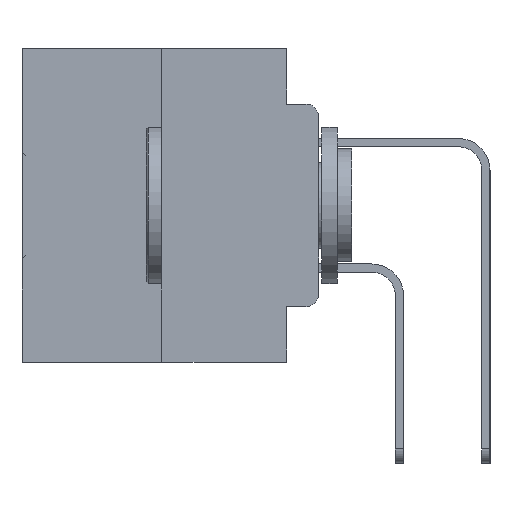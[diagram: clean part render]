
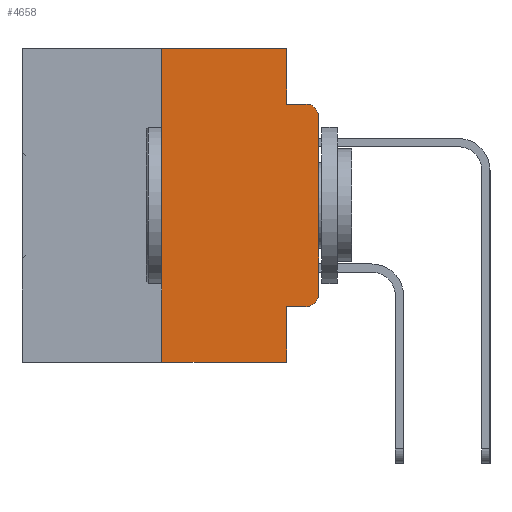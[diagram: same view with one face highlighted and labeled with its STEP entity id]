
A CAD part, left-side view. The second image highlights one B-rep face of the part: STEP entity #4658.
In plain terms, the highlighted planar face has unit normal (-1, 0, 0).
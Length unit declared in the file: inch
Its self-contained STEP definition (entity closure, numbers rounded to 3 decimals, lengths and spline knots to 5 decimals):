
#190 = CARTESIAN_POINT ( 'NONE',  ( 0., 0.473, 0. ) ) ;
#688 = LINE ( 'NONE', #13337, #14145 ) ;
#1972 = EDGE_CURVE ( 'NONE', #3401, #3729, #688, .T. ) ;
#2183 = FACE_OUTER_BOUND ( 'NONE', #27340, .T. ) ;
#2948 = VECTOR ( 'NONE', #24054, 39.37008 ) ;
#3268 = VECTOR ( 'NONE', #16422, 39.37008 ) ;
#3401 = VERTEX_POINT ( 'NONE', #32693 ) ;
#3729 = VERTEX_POINT ( 'NONE', #21136 ) ;
#3745 = DIRECTION ( 'NONE',  ( -1., 0., 0. ) ) ;
#3800 = ORIENTED_EDGE ( 'NONE', *, *, #30094, .T. ) ;
#3919 = CARTESIAN_POINT ( 'NONE',  ( 0., 0.051, -0.4115 ) ) ;
#4105 = AXIS2_PLACEMENT_3D ( 'NONE', #19871, #3745, #22589 ) ;
#4202 = CARTESIAN_POINT ( 'NONE',  ( 0., 0., 0. ) ) ;
#4546 = DIRECTION ( 'NONE',  ( 0., 0., -1. ) ) ;
#4658 = ADVANCED_FACE ( 'NONE', ( #2183 ), #17937, .F. ) ;
#5143 = VERTEX_POINT ( 'NONE', #3919 ) ;
#5626 = CARTESIAN_POINT ( 'NONE',  ( 0., 0.02, -0.4115 ) ) ;
#5742 = EDGE_CURVE ( 'NONE', #5143, #10630, #19257, .T. ) ;
#6447 = LINE ( 'NONE', #190, #11897 ) ;
#6921 = DIRECTION ( 'NONE',  ( 0., 0., 1. ) ) ;
#8018 = ORIENTED_EDGE ( 'NONE', *, *, #17838, .F. ) ;
#8147 = AXIS2_PLACEMENT_3D ( 'NONE', #10281, #29152, #12981 ) ;
#8456 = ORIENTED_EDGE ( 'NONE', *, *, #1972, .F. ) ;
#8635 = CARTESIAN_POINT ( 'NONE',  ( 0., 0.02, -0.0885 ) ) ;
#8859 = VERTEX_POINT ( 'NONE', #20877 ) ;
#8885 = ORIENTED_EDGE ( 'NONE', *, *, #33506, .T. ) ;
#8962 = CARTESIAN_POINT ( 'NONE',  ( 0., 0., -0.3915 ) ) ;
#9283 = EDGE_CURVE ( 'NONE', #5143, #31041, #29585, .T. ) ;
#10090 = LINE ( 'NONE', #34733, #2948 ) ;
#10281 = CARTESIAN_POINT ( 'NONE',  ( 0., 0.02, -0.1085 ) ) ;
#10304 = CARTESIAN_POINT ( 'NONE',  ( 0., 0.051, -0.5 ) ) ;
#10630 = VERTEX_POINT ( 'NONE', #5626 ) ;
#10942 = ORIENTED_EDGE ( 'NONE', *, *, #29273, .T. ) ;
#11369 = ORIENTED_EDGE ( 'NONE', *, *, #27605, .F. ) ;
#11425 = VERTEX_POINT ( 'NONE', #8635 ) ;
#11897 = VECTOR ( 'NONE', #24332, 39.37008 ) ;
#12510 = CARTESIAN_POINT ( 'NONE',  ( 0., 0.473, 0. ) ) ;
#12641 = ORIENTED_EDGE ( 'NONE', *, *, #5742, .T. ) ;
#12981 = DIRECTION ( 'NONE',  ( 0., 0., -1. ) ) ;
#13337 = CARTESIAN_POINT ( 'NONE',  ( 0., 0.25, 0. ) ) ;
#14145 = VECTOR ( 'NONE', #21501, 39.37008 ) ;
#14275 = LINE ( 'NONE', #4202, #27804 ) ;
#14323 = DIRECTION ( 'NONE',  ( 0., -1., 0. ) ) ;
#14712 = CARTESIAN_POINT ( 'NONE',  ( 0., 0.051, 0. ) ) ;
#14745 = CIRCLE ( 'NONE', #8147, 0.02 ) ;
#15294 = EDGE_CURVE ( 'NONE', #34616, #11425, #14745, .T. ) ;
#16422 = DIRECTION ( 'NONE',  ( 0., 0., -1. ) ) ;
#16773 = DIRECTION ( 'NONE',  ( 0., -1., 0. ) ) ;
#16827 = ORIENTED_EDGE ( 'NONE', *, *, #33002, .F. ) ;
#16978 = CARTESIAN_POINT ( 'NONE',  ( 0., 0., -0.1085 ) ) ;
#17838 = EDGE_CURVE ( 'NONE', #32907, #11425, #28985, .T. ) ;
#17937 = PLANE ( 'NONE',  #30563 ) ;
#19257 = LINE ( 'NONE', #27789, #25578 ) ;
#19871 = CARTESIAN_POINT ( 'NONE',  ( 0., 0.02, -0.3915 ) ) ;
#20661 = DIRECTION ( 'NONE',  ( 1., 0., 0. ) ) ;
#20877 = CARTESIAN_POINT ( 'NONE',  ( 0., 0.051, 0. ) ) ;
#21136 = CARTESIAN_POINT ( 'NONE',  ( 0., 0.25, 0. ) ) ;
#21260 = CARTESIAN_POINT ( 'NONE',  ( 0., 0.051, -0.0885 ) ) ;
#21501 = DIRECTION ( 'NONE',  ( 0., 0., 1. ) ) ;
#22589 = DIRECTION ( 'NONE',  ( 0., 0., -1. ) ) ;
#22642 = VECTOR ( 'NONE', #16773, 39.37008 ) ;
#23908 = LINE ( 'NONE', #32562, #3268 ) ;
#24054 = DIRECTION ( 'NONE',  ( 0., -1., 0. ) ) ;
#24332 = DIRECTION ( 'NONE',  ( 0., -1., 0. ) ) ;
#25578 = VECTOR ( 'NONE', #14323, 39.37008 ) ;
#27340 = EDGE_LOOP ( 'NONE', ( #10942, #33253, #8018, #16827, #11369, #8456, #3800, #33282, #12641, #8885 ) ) ;
#27605 = EDGE_CURVE ( 'NONE', #3729, #8859, #6447, .T. ) ;
#27789 = CARTESIAN_POINT ( 'NONE',  ( 0., 0.051, -0.4115 ) ) ;
#27804 = VECTOR ( 'NONE', #6921, 39.37008 ) ;
#28738 = VECTOR ( 'NONE', #30875, 39.37008 ) ;
#28919 = VERTEX_POINT ( 'NONE', #8962 ) ;
#28985 = LINE ( 'NONE', #32908, #22642 ) ;
#29152 = DIRECTION ( 'NONE',  ( -1., 0., 0. ) ) ;
#29273 = EDGE_CURVE ( 'NONE', #28919, #34616, #14275, .T. ) ;
#29382 = CIRCLE ( 'NONE', #4105, 0.02 ) ;
#29585 = LINE ( 'NONE', #14712, #28738 ) ;
#30094 = EDGE_CURVE ( 'NONE', #3401, #31041, #10090, .T. ) ;
#30563 = AXIS2_PLACEMENT_3D ( 'NONE', #12510, #20661, #4546 ) ;
#30875 = DIRECTION ( 'NONE',  ( 0., 0., -1. ) ) ;
#31041 = VERTEX_POINT ( 'NONE', #10304 ) ;
#32562 = CARTESIAN_POINT ( 'NONE',  ( 0., 0.051, 0. ) ) ;
#32693 = CARTESIAN_POINT ( 'NONE',  ( 0., 0.25, -0.5 ) ) ;
#32907 = VERTEX_POINT ( 'NONE', #21260 ) ;
#32908 = CARTESIAN_POINT ( 'NONE',  ( 0., 0.051, -0.0885 ) ) ;
#33002 = EDGE_CURVE ( 'NONE', #8859, #32907, #23908, .T. ) ;
#33253 = ORIENTED_EDGE ( 'NONE', *, *, #15294, .T. ) ;
#33282 = ORIENTED_EDGE ( 'NONE', *, *, #9283, .F. ) ;
#33506 = EDGE_CURVE ( 'NONE', #10630, #28919, #29382, .T. ) ;
#34616 = VERTEX_POINT ( 'NONE', #16978 ) ;
#34733 = CARTESIAN_POINT ( 'NONE',  ( 0., 0.473, -0.5 ) ) ;
